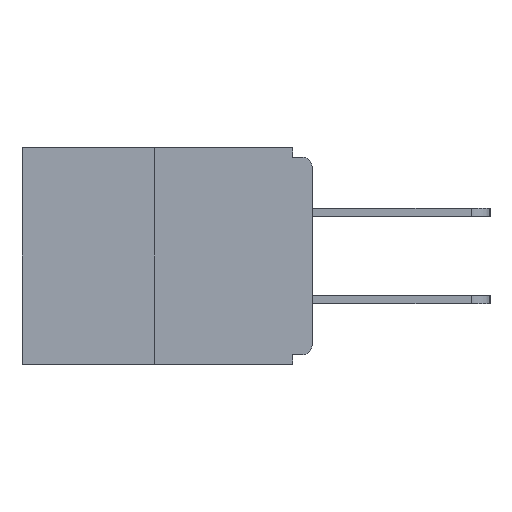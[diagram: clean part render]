
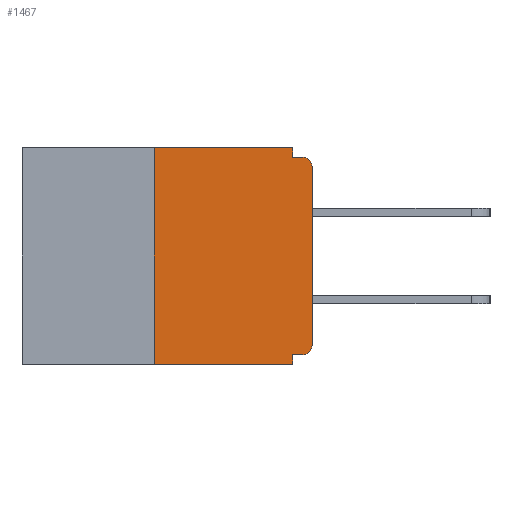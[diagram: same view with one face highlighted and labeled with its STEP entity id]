
A CAD part, left-side view. The second image highlights one B-rep face of the part: STEP entity #1467.
In plain terms, the highlighted planar face has unit normal (-1, 0, 0).
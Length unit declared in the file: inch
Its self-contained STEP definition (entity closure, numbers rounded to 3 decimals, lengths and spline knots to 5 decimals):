
#55 = DIRECTION ( 'NONE',  ( 0., 0., -1. ) ) ;
#90 = EDGE_CURVE ( 'NONE', #10953, #19196, #13112, .T. ) ;
#249 = ORIENTED_EDGE ( 'NONE', *, *, #18866, .T. ) ;
#289 = VECTOR ( 'NONE', #1845, 39.37008 ) ;
#320 = VERTEX_POINT ( 'NONE', #19522 ) ;
#480 = PLANE ( 'NONE',  #10544 ) ;
#688 = EDGE_CURVE ( 'NONE', #11888, #4062, #4387, .T. ) ;
#1015 = CARTESIAN_POINT ( 'NONE',  ( 0., 0.031, -0.328 ) ) ;
#1467 = ADVANCED_FACE ( 'NONE', ( #14703 ), #480, .F. ) ;
#1478 = DIRECTION ( 'NONE',  ( 0., -1., 0. ) ) ;
#1845 = DIRECTION ( 'NONE',  ( 0., 1., 0. ) ) ;
#2319 = LINE ( 'NONE', #14508, #17863 ) ;
#2449 = ORIENTED_EDGE ( 'NONE', *, *, #10466, .F. ) ;
#2923 = EDGE_CURVE ( 'NONE', #4062, #15625, #9762, .T. ) ;
#3075 = CARTESIAN_POINT ( 'NONE',  ( 0., 0.015, -0.03 ) ) ;
#3110 = ORIENTED_EDGE ( 'NONE', *, *, #90, .F. ) ;
#3859 = VECTOR ( 'NONE', #12871, 39.37008 ) ;
#4062 = VERTEX_POINT ( 'NONE', #16033 ) ;
#4137 = CARTESIAN_POINT ( 'NONE',  ( 0., 0.46, 0. ) ) ;
#4387 = LINE ( 'NONE', #15076, #7464 ) ;
#4546 = LINE ( 'NONE', #12083, #14630 ) ;
#5286 = CARTESIAN_POINT ( 'NONE',  ( 0., 0.031, 0. ) ) ;
#5290 = EDGE_CURVE ( 'NONE', #10739, #320, #18244, .T. ) ;
#5318 = DIRECTION ( 'NONE',  ( 0., 0., 1. ) ) ;
#5663 = VERTEX_POINT ( 'NONE', #13421 ) ;
#5750 = CARTESIAN_POINT ( 'NONE',  ( 0., 0., -0.313 ) ) ;
#6307 = DIRECTION ( 'NONE',  ( -1., 0., 0. ) ) ;
#6366 = ORIENTED_EDGE ( 'NONE', *, *, #5290, .T. ) ;
#6500 = CARTESIAN_POINT ( 'NONE',  ( 0., 0.46, 0. ) ) ;
#6849 = LINE ( 'NONE', #16170, #19101 ) ;
#7464 = VECTOR ( 'NONE', #5318, 39.37008 ) ;
#7907 = DIRECTION ( 'NONE',  ( 0., 0., -1. ) ) ;
#8002 = ORIENTED_EDGE ( 'NONE', *, *, #2923, .F. ) ;
#8258 = ORIENTED_EDGE ( 'NONE', *, *, #688, .F. ) ;
#8620 = ORIENTED_EDGE ( 'NONE', *, *, #11539, .T. ) ;
#9539 = DIRECTION ( 'NONE',  ( 0., 0., -1. ) ) ;
#9622 = VECTOR ( 'NONE', #13295, 39.37008 ) ;
#9762 = LINE ( 'NONE', #4137, #3859 ) ;
#10466 = EDGE_CURVE ( 'NONE', #15625, #5663, #4546, .T. ) ;
#10544 = AXIS2_PLACEMENT_3D ( 'NONE', #6500, #17278, #9539 ) ;
#10646 = EDGE_CURVE ( 'NONE', #11888, #19196, #6849, .T. ) ;
#10739 = VERTEX_POINT ( 'NONE', #14819 ) ;
#10751 = VECTOR ( 'NONE', #1478, 39.37008 ) ;
#10800 = VERTEX_POINT ( 'NONE', #5750 ) ;
#10953 = VERTEX_POINT ( 'NONE', #1015 ) ;
#11142 = CARTESIAN_POINT ( 'NONE',  ( 0., 0.015, -0.313 ) ) ;
#11391 = LINE ( 'NONE', #13664, #289 ) ;
#11539 = EDGE_CURVE ( 'NONE', #10800, #10739, #2319, .T. ) ;
#11888 = VERTEX_POINT ( 'NONE', #14202 ) ;
#11927 = CARTESIAN_POINT ( 'NONE',  ( 0., 0.015, -0.328 ) ) ;
#12083 = CARTESIAN_POINT ( 'NONE',  ( 0., 0.031, 0. ) ) ;
#12642 = EDGE_CURVE ( 'NONE', #5663, #320, #17810, .T. ) ;
#12871 = DIRECTION ( 'NONE',  ( 0., -1., 0. ) ) ;
#12881 = ORIENTED_EDGE ( 'NONE', *, *, #10646, .T. ) ;
#13112 = LINE ( 'NONE', #16415, #9622 ) ;
#13295 = DIRECTION ( 'NONE',  ( 0., 0., -1. ) ) ;
#13421 = CARTESIAN_POINT ( 'NONE',  ( 0., 0.031, -0.015 ) ) ;
#13664 = CARTESIAN_POINT ( 'NONE',  ( 0., 0., -0.328 ) ) ;
#13970 = CIRCLE ( 'NONE', #14989, 0.015 ) ;
#14202 = CARTESIAN_POINT ( 'NONE',  ( 0., 0.25, -0.343 ) ) ;
#14250 = EDGE_CURVE ( 'NONE', #18254, #10953, #11391, .T. ) ;
#14508 = CARTESIAN_POINT ( 'NONE',  ( 0., 0., 0. ) ) ;
#14587 = DIRECTION ( 'NONE',  ( 0., 0., -1. ) ) ;
#14630 = VECTOR ( 'NONE', #14587, 39.37008 ) ;
#14703 = FACE_OUTER_BOUND ( 'NONE', #19281, .T. ) ;
#14819 = CARTESIAN_POINT ( 'NONE',  ( 0., 0., -0.03 ) ) ;
#14989 = AXIS2_PLACEMENT_3D ( 'NONE', #11142, #16923, #7907 ) ;
#15032 = CARTESIAN_POINT ( 'NONE',  ( 0., 0.031, -0.343 ) ) ;
#15039 = CARTESIAN_POINT ( 'NONE',  ( 0., 0., -0.015 ) ) ;
#15076 = CARTESIAN_POINT ( 'NONE',  ( 0., 0.25, 0. ) ) ;
#15625 = VERTEX_POINT ( 'NONE', #5286 ) ;
#15792 = ORIENTED_EDGE ( 'NONE', *, *, #12642, .F. ) ;
#16033 = CARTESIAN_POINT ( 'NONE',  ( 0., 0.25, 0. ) ) ;
#16170 = CARTESIAN_POINT ( 'NONE',  ( 0., 0.46, -0.343 ) ) ;
#16415 = CARTESIAN_POINT ( 'NONE',  ( 0., 0.031, -0.343 ) ) ;
#16923 = DIRECTION ( 'NONE',  ( -1., 0., 0. ) ) ;
#17018 = AXIS2_PLACEMENT_3D ( 'NONE', #3075, #6307, #55 ) ;
#17278 = DIRECTION ( 'NONE',  ( 1., 0., 0. ) ) ;
#17681 = DIRECTION ( 'NONE',  ( 0., -1., 0. ) ) ;
#17742 = DIRECTION ( 'NONE',  ( 0., 0., 1. ) ) ;
#17810 = LINE ( 'NONE', #15039, #10751 ) ;
#17863 = VECTOR ( 'NONE', #17742, 39.37008 ) ;
#18244 = CIRCLE ( 'NONE', #17018, 0.015 ) ;
#18254 = VERTEX_POINT ( 'NONE', #11927 ) ;
#18866 = EDGE_CURVE ( 'NONE', #18254, #10800, #13970, .T. ) ;
#18971 = ORIENTED_EDGE ( 'NONE', *, *, #14250, .F. ) ;
#19101 = VECTOR ( 'NONE', #17681, 39.37008 ) ;
#19196 = VERTEX_POINT ( 'NONE', #15032 ) ;
#19281 = EDGE_LOOP ( 'NONE', ( #8002, #8258, #12881, #3110, #18971, #249, #8620, #6366, #15792, #2449 ) ) ;
#19522 = CARTESIAN_POINT ( 'NONE',  ( 0., 0.015, -0.015 ) ) ;
